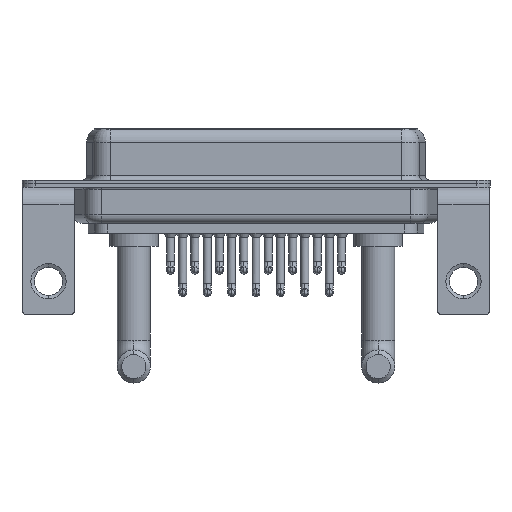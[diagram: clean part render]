
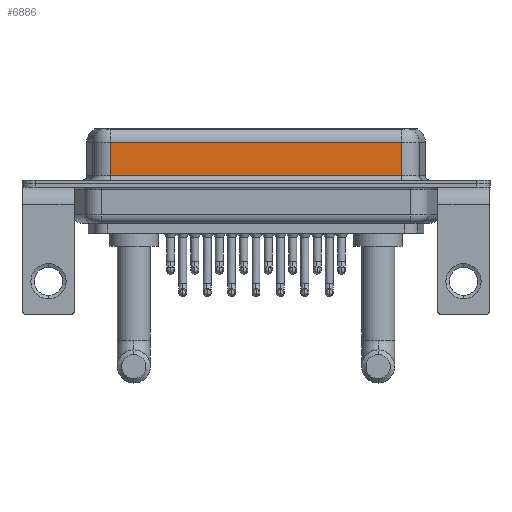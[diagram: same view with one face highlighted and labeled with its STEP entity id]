
A CAD part, front view. The second image highlights one B-rep face of the part: STEP entity #6886.
In plain terms, the highlighted planar face has unit normal (0, -1, 0).
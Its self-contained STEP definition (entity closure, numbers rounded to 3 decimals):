
#663 = EDGE_CURVE ( 'NONE', #20640, #10910, #5642, .T. ) ;
#1594 = DIRECTION ( 'NONE',  ( 0., 0., 1. ) ) ;
#1824 = CARTESIAN_POINT ( 'NONE',  ( 40.037, -3.95, 6.4 ) ) ;
#2272 = EDGE_LOOP ( 'NONE', ( #11876, #20327, #8086, #11603 ) ) ;
#3342 = VECTOR ( 'NONE', #5855, 1000. ) ;
#3455 = FACE_OUTER_BOUND ( 'NONE', #2272, .T. ) ;
#4105 = EDGE_CURVE ( 'NONE', #10910, #12508, #11230, .T. ) ;
#5070 = DIRECTION ( 'NONE',  ( 0., 0., -1. ) ) ;
#5642 = LINE ( 'NONE', #12338, #3342 ) ;
#5855 = DIRECTION ( 'NONE',  ( -1., 0., 0. ) ) ;
#6702 = EDGE_CURVE ( 'NONE', #12508, #6728, #11427, .T. ) ;
#6728 = VERTEX_POINT ( 'NONE', #14817 ) ;
#6886 = ADVANCED_FACE ( 'NONE', ( #3455 ), #16685, .F. ) ;
#7780 = AXIS2_PLACEMENT_3D ( 'NONE', #1824, #9932, #1594 ) ;
#8086 = ORIENTED_EDGE ( 'NONE', *, *, #4105, .T. ) ;
#8260 = CARTESIAN_POINT ( 'NONE',  ( 7.013, -3.95, 6.4 ) ) ;
#9800 = DIRECTION ( 'NONE',  ( 0., 0., -1. ) ) ;
#9932 = DIRECTION ( 'NONE',  ( 0., 1., 0. ) ) ;
#10566 = CARTESIAN_POINT ( 'NONE',  ( 40.037, -3.95, 4.65 ) ) ;
#10910 = VERTEX_POINT ( 'NONE', #15681 ) ;
#11230 = LINE ( 'NONE', #8260, #14670 ) ;
#11427 = LINE ( 'NONE', #11532, #12356 ) ;
#11532 = CARTESIAN_POINT ( 'NONE',  ( 40.037, -3.95, 0.9 ) ) ;
#11603 = ORIENTED_EDGE ( 'NONE', *, *, #6702, .T. ) ;
#11876 = ORIENTED_EDGE ( 'NONE', *, *, #15467, .F. ) ;
#12338 = CARTESIAN_POINT ( 'NONE',  ( 40.037, -3.95, 4.65 ) ) ;
#12356 = VECTOR ( 'NONE', #18080, 1000. ) ;
#12508 = VERTEX_POINT ( 'NONE', #16424 ) ;
#14670 = VECTOR ( 'NONE', #9800, 1000. ) ;
#14817 = CARTESIAN_POINT ( 'NONE',  ( 40.037, -3.95, 0.9 ) ) ;
#15467 = EDGE_CURVE ( 'NONE', #20640, #6728, #18510, .T. ) ;
#15681 = CARTESIAN_POINT ( 'NONE',  ( 7.013, -3.95, 4.65 ) ) ;
#16424 = CARTESIAN_POINT ( 'NONE',  ( 7.013, -3.95, 0.9 ) ) ;
#16685 = PLANE ( 'NONE',  #7780 ) ;
#16761 = CARTESIAN_POINT ( 'NONE',  ( 40.037, -3.95, 6.4 ) ) ;
#18080 = DIRECTION ( 'NONE',  ( 1., 0., 0. ) ) ;
#18510 = LINE ( 'NONE', #16761, #20829 ) ;
#20327 = ORIENTED_EDGE ( 'NONE', *, *, #663, .T. ) ;
#20640 = VERTEX_POINT ( 'NONE', #10566 ) ;
#20829 = VECTOR ( 'NONE', #5070, 1000. ) ;
